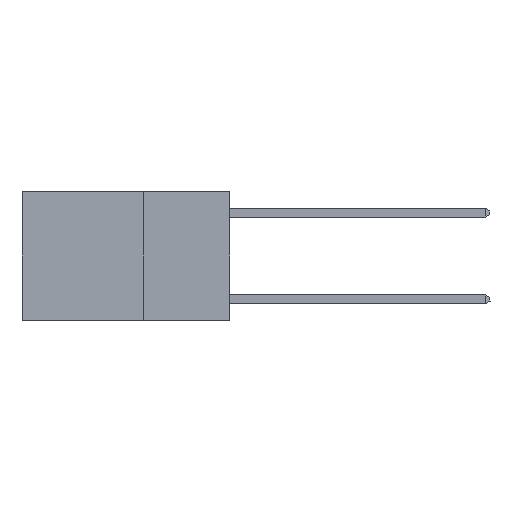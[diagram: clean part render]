
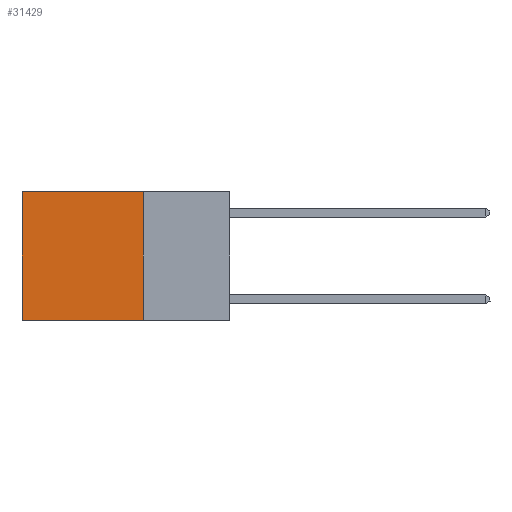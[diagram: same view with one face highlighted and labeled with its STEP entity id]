
A CAD part, left-side view. The second image highlights one B-rep face of the part: STEP entity #31429.
In plain terms, the highlighted planar face has unit normal (-1, 0, 0).
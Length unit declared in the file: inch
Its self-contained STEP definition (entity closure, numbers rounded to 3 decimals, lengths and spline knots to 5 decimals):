
#444 = VERTEX_POINT ( 'NONE', #3780 ) ;
#474 = ORIENTED_EDGE ( 'NONE', *, *, #2855, .F. ) ;
#2855 = EDGE_CURVE ( 'NONE', #3901, #444, #14897, .T. ) ;
#3780 = CARTESIAN_POINT ( 'NONE',  ( 0.2625, 0.25, -0.37 ) ) ;
#3901 = VERTEX_POINT ( 'NONE', #25237 ) ;
#4055 = VERTEX_POINT ( 'NONE', #16128 ) ;
#4365 = CARTESIAN_POINT ( 'NONE',  ( 0.2625, 0.25, 0. ) ) ;
#5207 = VECTOR ( 'NONE', #10263, 39.37008 ) ;
#6835 = LINE ( 'NONE', #22320, #5207 ) ;
#10263 = DIRECTION ( 'NONE',  ( 0., 0., -1. ) ) ;
#11464 = CARTESIAN_POINT ( 'NONE',  ( 0.2625, 0.25, 0. ) ) ;
#12003 = VECTOR ( 'NONE', #23939, 39.37008 ) ;
#12139 = ORIENTED_EDGE ( 'NONE', *, *, #26607, .T. ) ;
#13640 = EDGE_LOOP ( 'NONE', ( #19231, #24526, #474, #12139 ) ) ;
#13869 = CARTESIAN_POINT ( 'NONE',  ( 0.2625, 0.6, -0.37 ) ) ;
#13914 = DIRECTION ( 'NONE',  ( 0., 0., -1. ) ) ;
#14897 = LINE ( 'NONE', #21345, #26880 ) ;
#16128 = CARTESIAN_POINT ( 'NONE',  ( 0.2625, 0.6, 0. ) ) ;
#18252 = LINE ( 'NONE', #19492, #30216 ) ;
#18284 = AXIS2_PLACEMENT_3D ( 'NONE', #11464, #28263, #13914 ) ;
#19231 = ORIENTED_EDGE ( 'NONE', *, *, #28100, .T. ) ;
#19492 = CARTESIAN_POINT ( 'NONE',  ( 0.2625, 0.25, -0.37 ) ) ;
#21345 = CARTESIAN_POINT ( 'NONE',  ( 0.2625, 0.25, 0. ) ) ;
#21497 = FACE_OUTER_BOUND ( 'NONE', #13640, .T. ) ;
#21879 = DIRECTION ( 'NONE',  ( 0., 1., 0. ) ) ;
#21885 = VERTEX_POINT ( 'NONE', #13869 ) ;
#22320 = CARTESIAN_POINT ( 'NONE',  ( 0.2625, 0.6, 0. ) ) ;
#23939 = DIRECTION ( 'NONE',  ( 0., 1., 0. ) ) ;
#24075 = LINE ( 'NONE', #4365, #12003 ) ;
#24084 = EDGE_CURVE ( 'NONE', #444, #21885, #18252, .T. ) ;
#24526 = ORIENTED_EDGE ( 'NONE', *, *, #24084, .F. ) ;
#25237 = CARTESIAN_POINT ( 'NONE',  ( 0.2625, 0.25, 0. ) ) ;
#25887 = PLANE ( 'NONE',  #18284 ) ;
#26607 = EDGE_CURVE ( 'NONE', #3901, #4055, #24075, .T. ) ;
#26880 = VECTOR ( 'NONE', #30948, 39.37008 ) ;
#28100 = EDGE_CURVE ( 'NONE', #4055, #21885, #6835, .T. ) ;
#28263 = DIRECTION ( 'NONE',  ( 1., 0., 0. ) ) ;
#30216 = VECTOR ( 'NONE', #21879, 39.37008 ) ;
#30948 = DIRECTION ( 'NONE',  ( 0., 0., -1. ) ) ;
#31429 = ADVANCED_FACE ( 'NONE', ( #21497 ), #25887, .F. ) ;
